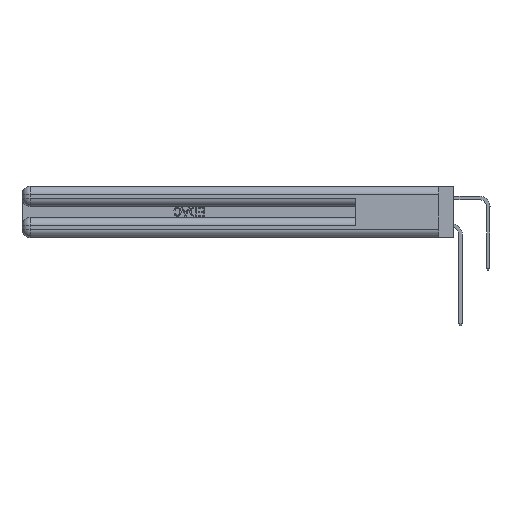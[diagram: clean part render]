
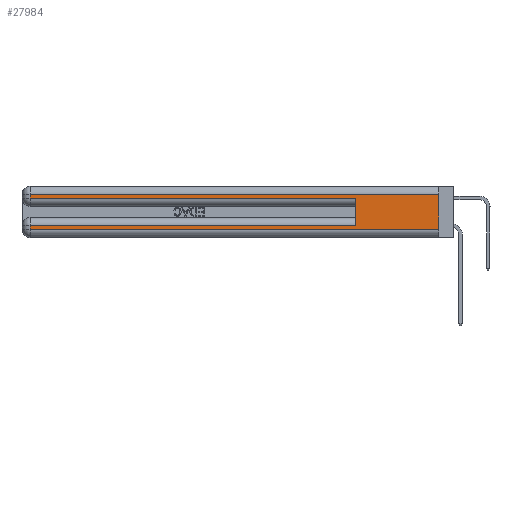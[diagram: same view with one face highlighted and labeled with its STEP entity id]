
A CAD part, left-side view. The second image highlights one B-rep face of the part: STEP entity #27984.
In plain terms, the highlighted planar face has unit normal (-1, 0, 0).
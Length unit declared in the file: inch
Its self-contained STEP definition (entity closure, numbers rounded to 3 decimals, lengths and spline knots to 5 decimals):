
#995 = VECTOR ( 'NONE', #12128, 39.37008 ) ;
#1139 = EDGE_CURVE ( 'NONE', #17568, #9824, #22401, .T. ) ;
#2841 = CARTESIAN_POINT ( 'NONE',  ( 0., 0., 0.06 ) ) ;
#3037 = CARTESIAN_POINT ( 'NONE',  ( 0., 0.6, 0.085 ) ) ;
#3518 = DIRECTION ( 'NONE',  ( 0., 0., 1. ) ) ;
#3613 = LINE ( 'NONE', #38157, #11893 ) ;
#4768 = CARTESIAN_POINT ( 'NONE',  ( 0., 0., 0.285 ) ) ;
#4844 = EDGE_CURVE ( 'NONE', #17568, #30229, #6076, .T. ) ;
#4990 = CARTESIAN_POINT ( 'NONE',  ( 0., 0., 0.31 ) ) ;
#5693 = EDGE_CURVE ( 'NONE', #14921, #38956, #32540, .T. ) ;
#6076 = LINE ( 'NONE', #4990, #15458 ) ;
#7256 = EDGE_CURVE ( 'NONE', #32342, #9824, #9087, .T. ) ;
#9087 = LINE ( 'NONE', #2841, #36801 ) ;
#9385 = ORIENTED_EDGE ( 'NONE', *, *, #18205, .T. ) ;
#9409 = DIRECTION ( 'NONE',  ( 0., 0., -1. ) ) ;
#9824 = VERTEX_POINT ( 'NONE', #26700 ) ;
#10892 = FACE_OUTER_BOUND ( 'NONE', #12140, .T. ) ;
#11647 = DIRECTION ( 'NONE',  ( 0., 1., 0. ) ) ;
#11893 = VECTOR ( 'NONE', #13481, 39.37008 ) ;
#12128 = DIRECTION ( 'NONE',  ( 0., 1., 0. ) ) ;
#12140 = EDGE_LOOP ( 'NONE', ( #33745, #41027, #9385, #15317, #35009, #23834, #31831, #16104 ) ) ;
#13137 = PLANE ( 'NONE',  #26127 ) ;
#13147 = EDGE_CURVE ( 'NONE', #17136, #32342, #3613, .T. ) ;
#13481 = DIRECTION ( 'NONE',  ( 0., 0., -1. ) ) ;
#14921 = VERTEX_POINT ( 'NONE', #17704 ) ;
#15317 = ORIENTED_EDGE ( 'NONE', *, *, #5693, .T. ) ;
#15458 = VECTOR ( 'NONE', #11647, 39.37008 ) ;
#16104 = ORIENTED_EDGE ( 'NONE', *, *, #7256, .T. ) ;
#16477 = LINE ( 'NONE', #29802, #995 ) ;
#16954 = CARTESIAN_POINT ( 'NONE',  ( 0., 2.94, 0.31 ) ) ;
#17136 = VERTEX_POINT ( 'NONE', #26703 ) ;
#17568 = VERTEX_POINT ( 'NONE', #24570 ) ;
#17704 = CARTESIAN_POINT ( 'NONE',  ( 0., 2.94, 0.285 ) ) ;
#18205 = EDGE_CURVE ( 'NONE', #30229, #14921, #24560, .T. ) ;
#19073 = EDGE_CURVE ( 'NONE', #28573, #38956, #34550, .T. ) ;
#19151 = DIRECTION ( 'NONE',  ( 0., -1., 0. ) ) ;
#20203 = VECTOR ( 'NONE', #34819, 39.37008 ) ;
#22401 = LINE ( 'NONE', #38082, #20203 ) ;
#23816 = DIRECTION ( 'NONE',  ( 1., 0., 0. ) ) ;
#23834 = ORIENTED_EDGE ( 'NONE', *, *, #43735, .T. ) ;
#24560 = LINE ( 'NONE', #37878, #28444 ) ;
#24570 = CARTESIAN_POINT ( 'NONE',  ( 0., 0., 0.31 ) ) ;
#26127 = AXIS2_PLACEMENT_3D ( 'NONE', #27084, #23816, #9409 ) ;
#26700 = CARTESIAN_POINT ( 'NONE',  ( 0., 0., 0.06 ) ) ;
#26703 = CARTESIAN_POINT ( 'NONE',  ( 0., 2.94, 0.085 ) ) ;
#27084 = CARTESIAN_POINT ( 'NONE',  ( 0., 0., 0.37 ) ) ;
#27863 = VECTOR ( 'NONE', #3518, 39.37008 ) ;
#27984 = ADVANCED_FACE ( 'NONE', ( #10892 ), #13137, .F. ) ;
#28444 = VECTOR ( 'NONE', #34009, 39.37008 ) ;
#28573 = VERTEX_POINT ( 'NONE', #3037 ) ;
#29802 = CARTESIAN_POINT ( 'NONE',  ( 0., 0., 0.085 ) ) ;
#30229 = VERTEX_POINT ( 'NONE', #16954 ) ;
#30921 = CARTESIAN_POINT ( 'NONE',  ( 0., 0.6, 0.285 ) ) ;
#31831 = ORIENTED_EDGE ( 'NONE', *, *, #13147, .T. ) ;
#32342 = VERTEX_POINT ( 'NONE', #36773 ) ;
#32540 = LINE ( 'NONE', #4768, #43636 ) ;
#33745 = ORIENTED_EDGE ( 'NONE', *, *, #1139, .F. ) ;
#34009 = DIRECTION ( 'NONE',  ( 0., 0., -1. ) ) ;
#34550 = LINE ( 'NONE', #45484, #27863 ) ;
#34819 = DIRECTION ( 'NONE',  ( 0., 0., -1. ) ) ;
#35009 = ORIENTED_EDGE ( 'NONE', *, *, #19073, .F. ) ;
#36773 = CARTESIAN_POINT ( 'NONE',  ( 0., 2.94, 0.06 ) ) ;
#36801 = VECTOR ( 'NONE', #44947, 39.37008 ) ;
#37878 = CARTESIAN_POINT ( 'NONE',  ( 0., 2.94, 0.37 ) ) ;
#38082 = CARTESIAN_POINT ( 'NONE',  ( 0., 0., 0.37 ) ) ;
#38157 = CARTESIAN_POINT ( 'NONE',  ( 0., 2.94, 0.37 ) ) ;
#38956 = VERTEX_POINT ( 'NONE', #30921 ) ;
#41027 = ORIENTED_EDGE ( 'NONE', *, *, #4844, .T. ) ;
#43636 = VECTOR ( 'NONE', #19151, 39.37008 ) ;
#43735 = EDGE_CURVE ( 'NONE', #28573, #17136, #16477, .T. ) ;
#44947 = DIRECTION ( 'NONE',  ( 0., -1., 0. ) ) ;
#45484 = CARTESIAN_POINT ( 'NONE',  ( 0., 0.6, 0.145 ) ) ;
